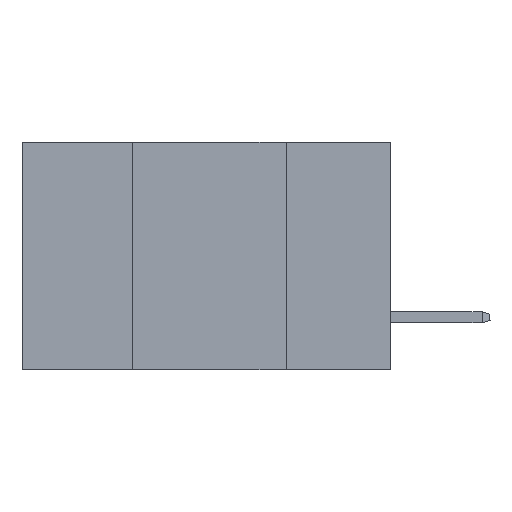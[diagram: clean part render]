
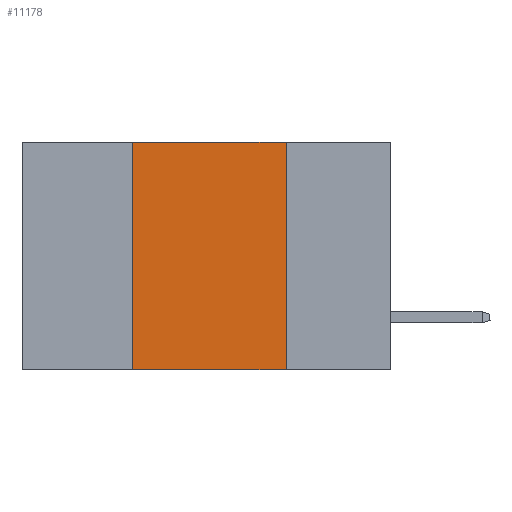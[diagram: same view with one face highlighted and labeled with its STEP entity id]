
A CAD part, left-side view. The second image highlights one B-rep face of the part: STEP entity #11178.
In plain terms, the highlighted planar face has unit normal (-1, 0, 0).
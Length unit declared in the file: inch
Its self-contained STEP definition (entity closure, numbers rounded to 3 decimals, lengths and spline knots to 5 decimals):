
#907 = DIRECTION ( 'NONE',  ( 1., 0., 0. ) ) ;
#2400 = EDGE_CURVE ( 'NONE', #8935, #11056, #9468, .T. ) ;
#3035 = VECTOR ( 'NONE', #12803, 39.37008 ) ;
#3680 = ORIENTED_EDGE ( 'NONE', *, *, #8915, .F. ) ;
#5502 = VECTOR ( 'NONE', #15422, 39.37008 ) ;
#5739 = CARTESIAN_POINT ( 'NONE',  ( 0., 0.6, 0. ) ) ;
#5743 = VECTOR ( 'NONE', #12793, 39.37008 ) ;
#6959 = DIRECTION ( 'NONE',  ( 0., -1., 0. ) ) ;
#7243 = EDGE_LOOP ( 'NONE', ( #3680, #9069, #10873, #12757 ) ) ;
#7498 = EDGE_CURVE ( 'NONE', #9697, #12543, #14754, .T. ) ;
#7809 = CARTESIAN_POINT ( 'NONE',  ( 0., 0.17, 0. ) ) ;
#8355 = AXIS2_PLACEMENT_3D ( 'NONE', #5739, #907, #9384 ) ;
#8915 = EDGE_CURVE ( 'NONE', #12543, #11056, #13150, .T. ) ;
#8935 = VERTEX_POINT ( 'NONE', #12569 ) ;
#9069 = ORIENTED_EDGE ( 'NONE', *, *, #7498, .F. ) ;
#9384 = DIRECTION ( 'NONE',  ( 0., 0., -1. ) ) ;
#9468 = LINE ( 'NONE', #12902, #3035 ) ;
#9697 = VERTEX_POINT ( 'NONE', #15088 ) ;
#10288 = FACE_OUTER_BOUND ( 'NONE', #7243, .T. ) ;
#10348 = CARTESIAN_POINT ( 'NONE',  ( 0., 0.17, -0.37 ) ) ;
#10660 = PLANE ( 'NONE',  #8355 ) ;
#10873 = ORIENTED_EDGE ( 'NONE', *, *, #11174, .F. ) ;
#11056 = VERTEX_POINT ( 'NONE', #10348 ) ;
#11174 = EDGE_CURVE ( 'NONE', #8935, #9697, #12721, .T. ) ;
#11178 = ADVANCED_FACE ( 'NONE', ( #10288 ), #10660, .F. ) ;
#12521 = CARTESIAN_POINT ( 'NONE',  ( 0., 0.17, 0. ) ) ;
#12543 = VERTEX_POINT ( 'NONE', #7809 ) ;
#12569 = CARTESIAN_POINT ( 'NONE',  ( 0., 0.42, -0.37 ) ) ;
#12721 = LINE ( 'NONE', #14091, #5502 ) ;
#12757 = ORIENTED_EDGE ( 'NONE', *, *, #2400, .T. ) ;
#12793 = DIRECTION ( 'NONE',  ( 0., 0., -1. ) ) ;
#12803 = DIRECTION ( 'NONE',  ( 0., -1., 0. ) ) ;
#12902 = CARTESIAN_POINT ( 'NONE',  ( 0., 0.6, -0.37 ) ) ;
#13150 = LINE ( 'NONE', #12521, #5743 ) ;
#14091 = CARTESIAN_POINT ( 'NONE',  ( 0., 0.42, 0. ) ) ;
#14179 = CARTESIAN_POINT ( 'NONE',  ( 0., 0.6, 0. ) ) ;
#14754 = LINE ( 'NONE', #14179, #14930 ) ;
#14930 = VECTOR ( 'NONE', #6959, 39.37008 ) ;
#15088 = CARTESIAN_POINT ( 'NONE',  ( 0., 0.42, 0. ) ) ;
#15422 = DIRECTION ( 'NONE',  ( 0., 0., 1. ) ) ;
